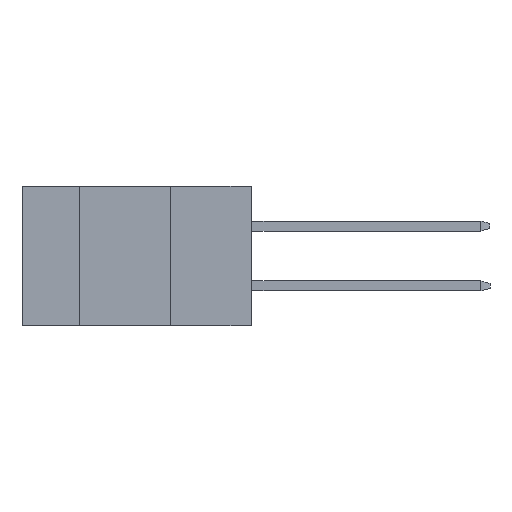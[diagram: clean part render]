
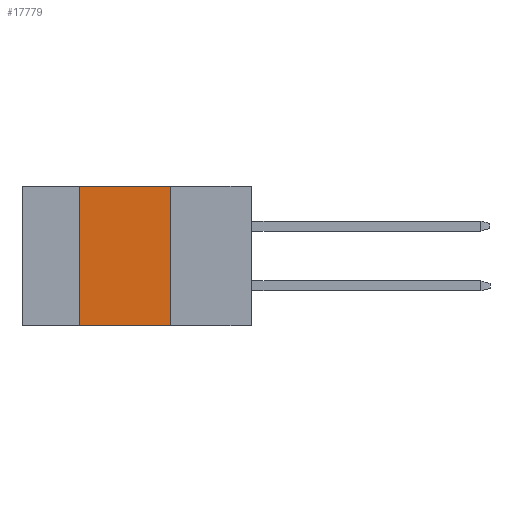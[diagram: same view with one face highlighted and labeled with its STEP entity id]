
A CAD part, left-side view. The second image highlights one B-rep face of the part: STEP entity #17779.
In plain terms, the highlighted planar face has unit normal (-1, 0, 0).
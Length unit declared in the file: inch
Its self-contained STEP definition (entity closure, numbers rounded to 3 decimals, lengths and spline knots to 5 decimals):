
#763 = AXIS2_PLACEMENT_3D ( 'NONE', #2446, #14042, #9755 ) ;
#1102 = VERTEX_POINT ( 'NONE', #18610 ) ;
#1171 = CARTESIAN_POINT ( 'NONE',  ( 0., 0.254, -0.437 ) ) ;
#1338 = ORIENTED_EDGE ( 'NONE', *, *, #16297, .F. ) ;
#1582 = VERTEX_POINT ( 'NONE', #13269 ) ;
#1626 = ORIENTED_EDGE ( 'NONE', *, *, #5142, .T. ) ;
#1665 = EDGE_CURVE ( 'NONE', #9092, #1102, #12206, .T. ) ;
#2446 = CARTESIAN_POINT ( 'NONE',  ( 0., 0.72, 0. ) ) ;
#2546 = ORIENTED_EDGE ( 'NONE', *, *, #14685, .F. ) ;
#2634 = LINE ( 'NONE', #15373, #5331 ) ;
#4004 = LINE ( 'NONE', #17219, #14649 ) ;
#4227 = VECTOR ( 'NONE', #9454, 39.37008 ) ;
#5142 = EDGE_CURVE ( 'NONE', #9092, #17836, #2634, .T. ) ;
#5331 = VECTOR ( 'NONE', #15650, 39.37008 ) ;
#5342 = CARTESIAN_POINT ( 'NONE',  ( 0., 0.54, -0.437 ) ) ;
#7075 = LINE ( 'NONE', #1171, #18310 ) ;
#7168 = DIRECTION ( 'NONE',  ( 0., 0., -1. ) ) ;
#8538 = CARTESIAN_POINT ( 'NONE',  ( 0., 0.254, -0.437 ) ) ;
#9092 = VERTEX_POINT ( 'NONE', #11274 ) ;
#9454 = DIRECTION ( 'NONE',  ( 0., 0., 1. ) ) ;
#9662 = PLANE ( 'NONE',  #763 ) ;
#9755 = DIRECTION ( 'NONE',  ( 0., 0., -1. ) ) ;
#11274 = CARTESIAN_POINT ( 'NONE',  ( 0., 0.54, -0.437 ) ) ;
#12206 = LINE ( 'NONE', #5342, #4227 ) ;
#12652 = EDGE_LOOP ( 'NONE', ( #1338, #2546, #15147, #1626 ) ) ;
#12665 = DIRECTION ( 'NONE',  ( 0., -1., 0. ) ) ;
#13269 = CARTESIAN_POINT ( 'NONE',  ( 0., 0.254, 0. ) ) ;
#14042 = DIRECTION ( 'NONE',  ( 1., 0., 0. ) ) ;
#14649 = VECTOR ( 'NONE', #12665, 39.37008 ) ;
#14685 = EDGE_CURVE ( 'NONE', #1102, #1582, #4004, .T. ) ;
#15147 = ORIENTED_EDGE ( 'NONE', *, *, #1665, .F. ) ;
#15373 = CARTESIAN_POINT ( 'NONE',  ( 0., 0.72, -0.437 ) ) ;
#15650 = DIRECTION ( 'NONE',  ( 0., -1., 0. ) ) ;
#16297 = EDGE_CURVE ( 'NONE', #1582, #17836, #7075, .T. ) ;
#17219 = CARTESIAN_POINT ( 'NONE',  ( 0., 0.72, 0. ) ) ;
#17779 = ADVANCED_FACE ( 'NONE', ( #18394 ), #9662, .F. ) ;
#17836 = VERTEX_POINT ( 'NONE', #8538 ) ;
#18310 = VECTOR ( 'NONE', #7168, 39.37008 ) ;
#18394 = FACE_OUTER_BOUND ( 'NONE', #12652, .T. ) ;
#18610 = CARTESIAN_POINT ( 'NONE',  ( 0., 0.54, 0. ) ) ;
